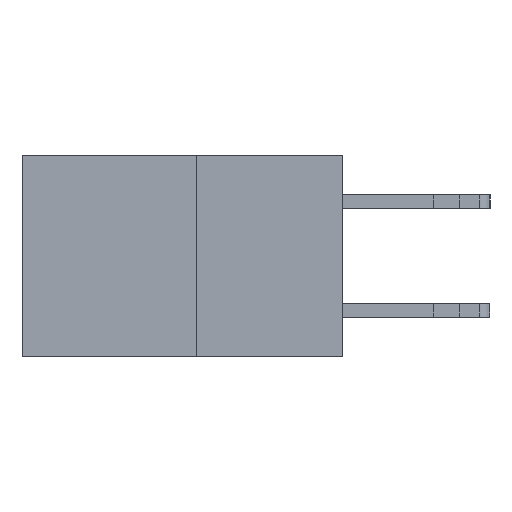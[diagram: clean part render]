
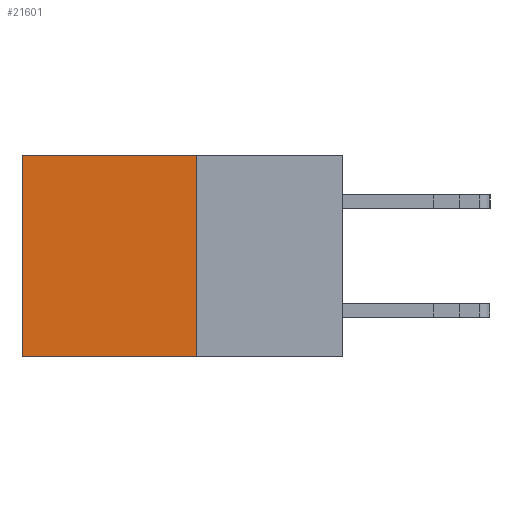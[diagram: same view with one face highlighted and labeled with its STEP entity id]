
A CAD part, left-side view. The second image highlights one B-rep face of the part: STEP entity #21601.
In plain terms, the highlighted planar face has unit normal (-1, 0, 0).
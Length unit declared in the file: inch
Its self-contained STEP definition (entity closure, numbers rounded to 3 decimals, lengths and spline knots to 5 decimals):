
#1042 = CARTESIAN_POINT ( 'NONE',  ( 0.277, 0.59, -0.37 ) ) ;
#1987 = LINE ( 'NONE', #3021, #17465 ) ;
#3021 = CARTESIAN_POINT ( 'NONE',  ( 0.277, 0.27, 0. ) ) ;
#3952 = ORIENTED_EDGE ( 'NONE', *, *, #11445, .T. ) ;
#4823 = EDGE_CURVE ( 'NONE', #18174, #14420, #13959, .T. ) ;
#6224 = PLANE ( 'NONE',  #11661 ) ;
#6282 = CARTESIAN_POINT ( 'NONE',  ( 0.277, 0.59, -0.37 ) ) ;
#6616 = VECTOR ( 'NONE', #23565, 39.37008 ) ;
#6813 = CARTESIAN_POINT ( 'NONE',  ( 0.277, 0.59, 0. ) ) ;
#6908 = CARTESIAN_POINT ( 'NONE',  ( 0.277, 0.27, -0.37 ) ) ;
#8250 = CARTESIAN_POINT ( 'NONE',  ( 0.277, 0.27, -0.37 ) ) ;
#8305 = DIRECTION ( 'NONE',  ( 0., 0., -1. ) ) ;
#8928 = DIRECTION ( 'NONE',  ( 0., 1., 0. ) ) ;
#8984 = EDGE_CURVE ( 'NONE', #13331, #24700, #23203, .T. ) ;
#9966 = EDGE_CURVE ( 'NONE', #24700, #14420, #10035, .T. ) ;
#10035 = LINE ( 'NONE', #6908, #20023 ) ;
#10259 = DIRECTION ( 'NONE',  ( 1., 0., 0. ) ) ;
#11445 = EDGE_CURVE ( 'NONE', #13331, #18174, #1987, .T. ) ;
#11661 = AXIS2_PLACEMENT_3D ( 'NONE', #8250, #10259, #24206 ) ;
#11963 = FACE_OUTER_BOUND ( 'NONE', #20228, .T. ) ;
#12805 = ORIENTED_EDGE ( 'NONE', *, *, #4823, .T. ) ;
#13313 = DIRECTION ( 'NONE',  ( 0., 1., 0. ) ) ;
#13331 = VERTEX_POINT ( 'NONE', #24680 ) ;
#13457 = ORIENTED_EDGE ( 'NONE', *, *, #9966, .F. ) ;
#13959 = LINE ( 'NONE', #6282, #24498 ) ;
#14420 = VERTEX_POINT ( 'NONE', #1042 ) ;
#17465 = VECTOR ( 'NONE', #13313, 39.37008 ) ;
#18174 = VERTEX_POINT ( 'NONE', #6813 ) ;
#20023 = VECTOR ( 'NONE', #8928, 39.37008 ) ;
#20228 = EDGE_LOOP ( 'NONE', ( #12805, #13457, #24628, #3952 ) ) ;
#21551 = CARTESIAN_POINT ( 'NONE',  ( 0.277, 0.27, -0.37 ) ) ;
#21601 = ADVANCED_FACE ( 'NONE', ( #11963 ), #6224, .F. ) ;
#23203 = LINE ( 'NONE', #21551, #6616 ) ;
#23565 = DIRECTION ( 'NONE',  ( 0., 0., -1. ) ) ;
#24206 = DIRECTION ( 'NONE',  ( 0., 0., -1. ) ) ;
#24498 = VECTOR ( 'NONE', #8305, 39.37008 ) ;
#24628 = ORIENTED_EDGE ( 'NONE', *, *, #8984, .F. ) ;
#24680 = CARTESIAN_POINT ( 'NONE',  ( 0.277, 0.27, 0. ) ) ;
#24700 = VERTEX_POINT ( 'NONE', #25413 ) ;
#25413 = CARTESIAN_POINT ( 'NONE',  ( 0.277, 0.27, -0.37 ) ) ;
